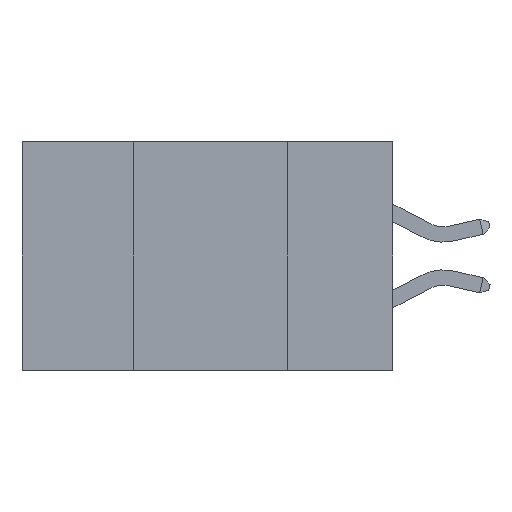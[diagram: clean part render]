
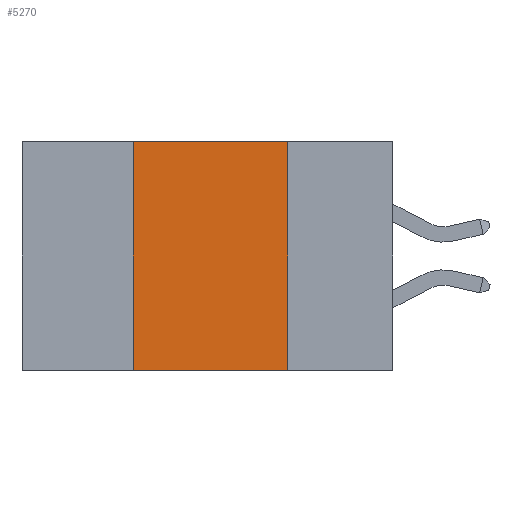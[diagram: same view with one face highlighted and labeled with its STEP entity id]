
A CAD part, left-side view. The second image highlights one B-rep face of the part: STEP entity #5270.
In plain terms, the highlighted planar face has unit normal (-1, 0, 0).
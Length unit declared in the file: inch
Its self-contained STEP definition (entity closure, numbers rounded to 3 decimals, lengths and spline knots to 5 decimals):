
#203 = ORIENTED_EDGE ( 'NONE', *, *, #781, .F. ) ;
#507 = CARTESIAN_POINT ( 'NONE',  ( 0., 0.42, -0.37 ) ) ;
#510 = CARTESIAN_POINT ( 'NONE',  ( 0., 0.17, 0. ) ) ;
#781 = EDGE_CURVE ( 'NONE', #13106, #13696, #4416, .T. ) ;
#782 = FACE_OUTER_BOUND ( 'NONE', #5848, .T. ) ;
#1334 = ORIENTED_EDGE ( 'NONE', *, *, #13197, .F. ) ;
#2526 = LINE ( 'NONE', #8890, #13105 ) ;
#2570 = ORIENTED_EDGE ( 'NONE', *, *, #7001, .T. ) ;
#2581 = DIRECTION ( 'NONE',  ( 0., 0., 1. ) ) ;
#3575 = CARTESIAN_POINT ( 'NONE',  ( 0., 0.17, -0.37 ) ) ;
#3988 = AXIS2_PLACEMENT_3D ( 'NONE', #14224, #5783, #9430 ) ;
#4416 = LINE ( 'NONE', #9763, #11757 ) ;
#4925 = EDGE_CURVE ( 'NONE', #13696, #6437, #2526, .T. ) ;
#5270 = ADVANCED_FACE ( 'NONE', ( #782 ), #9390, .F. ) ;
#5368 = CARTESIAN_POINT ( 'NONE',  ( 0., 0.6, -0.37 ) ) ;
#5689 = LINE ( 'NONE', #5368, #13615 ) ;
#5783 = DIRECTION ( 'NONE',  ( 1., 0., 0. ) ) ;
#5848 = EDGE_LOOP ( 'NONE', ( #1334, #14662, #203, #2570 ) ) ;
#6437 = VERTEX_POINT ( 'NONE', #510 ) ;
#7001 = EDGE_CURVE ( 'NONE', #13106, #13664, #5689, .T. ) ;
#8890 = CARTESIAN_POINT ( 'NONE',  ( 0., 0.6, 0. ) ) ;
#9390 = PLANE ( 'NONE',  #3988 ) ;
#9430 = DIRECTION ( 'NONE',  ( 0., 0., -1. ) ) ;
#9517 = LINE ( 'NONE', #13142, #13706 ) ;
#9763 = CARTESIAN_POINT ( 'NONE',  ( 0., 0.42, 0. ) ) ;
#10734 = CARTESIAN_POINT ( 'NONE',  ( 0., 0.42, 0. ) ) ;
#11757 = VECTOR ( 'NONE', #2581, 39.37008 ) ;
#11898 = DIRECTION ( 'NONE',  ( 0., 0., -1. ) ) ;
#13105 = VECTOR ( 'NONE', #13920, 39.37008 ) ;
#13106 = VERTEX_POINT ( 'NONE', #507 ) ;
#13142 = CARTESIAN_POINT ( 'NONE',  ( 0., 0.17, 0. ) ) ;
#13197 = EDGE_CURVE ( 'NONE', #6437, #13664, #9517, .T. ) ;
#13615 = VECTOR ( 'NONE', #15163, 39.37008 ) ;
#13664 = VERTEX_POINT ( 'NONE', #3575 ) ;
#13696 = VERTEX_POINT ( 'NONE', #10734 ) ;
#13706 = VECTOR ( 'NONE', #11898, 39.37008 ) ;
#13920 = DIRECTION ( 'NONE',  ( 0., -1., 0. ) ) ;
#14224 = CARTESIAN_POINT ( 'NONE',  ( 0., 0.6, 0. ) ) ;
#14662 = ORIENTED_EDGE ( 'NONE', *, *, #4925, .F. ) ;
#15163 = DIRECTION ( 'NONE',  ( 0., -1., 0. ) ) ;
